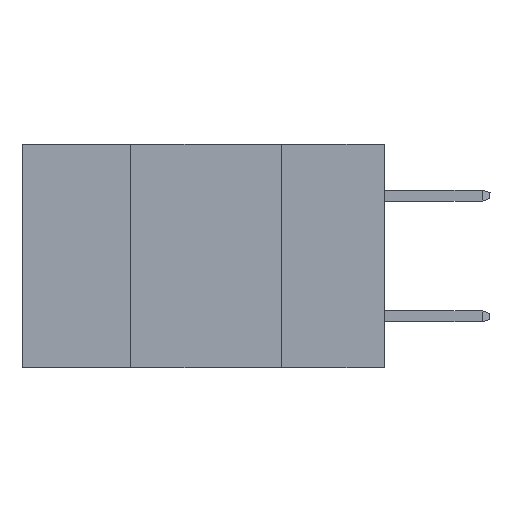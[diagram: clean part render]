
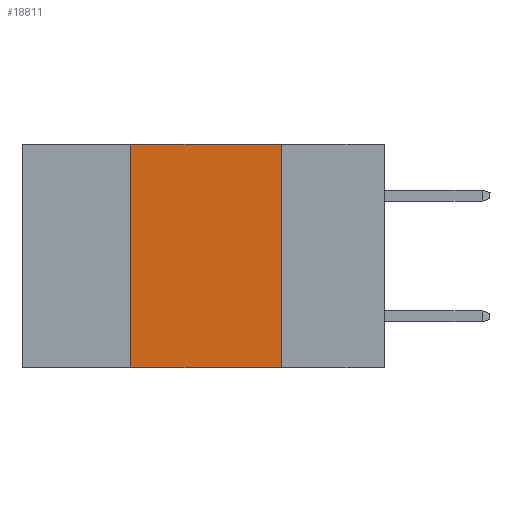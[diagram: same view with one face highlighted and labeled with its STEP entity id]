
A CAD part, left-side view. The second image highlights one B-rep face of the part: STEP entity #18811.
In plain terms, the highlighted planar face has unit normal (-1, 0, 0).
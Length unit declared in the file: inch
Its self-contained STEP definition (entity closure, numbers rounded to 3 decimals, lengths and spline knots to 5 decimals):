
#59 = ORIENTED_EDGE ( 'NONE', *, *, #3938, .T. ) ;
#1179 = CARTESIAN_POINT ( 'NONE',  ( 0., 0.42, -0.37 ) ) ;
#1969 = EDGE_CURVE ( 'NONE', #14255, #6165, #17362, .T. ) ;
#2814 = CARTESIAN_POINT ( 'NONE',  ( 0., 0.17, -0.37 ) ) ;
#3074 = EDGE_LOOP ( 'NONE', ( #12767, #3984, #19502, #59 ) ) ;
#3472 = CARTESIAN_POINT ( 'NONE',  ( 0., 0.42, 0. ) ) ;
#3938 = EDGE_CURVE ( 'NONE', #10778, #6165, #16680, .T. ) ;
#3984 = ORIENTED_EDGE ( 'NONE', *, *, #18024, .F. ) ;
#4234 = CARTESIAN_POINT ( 'NONE',  ( 0., 0.42, -0.37 ) ) ;
#4297 = LINE ( 'NONE', #8624, #9271 ) ;
#5072 = CARTESIAN_POINT ( 'NONE',  ( 0., 0.6, 0. ) ) ;
#5873 = DIRECTION ( 'NONE',  ( 0., 0., -1. ) ) ;
#6165 = VERTEX_POINT ( 'NONE', #2814 ) ;
#6980 = DIRECTION ( 'NONE',  ( 0., 0., -1. ) ) ;
#7395 = CARTESIAN_POINT ( 'NONE',  ( 0., 0.17, -0.37 ) ) ;
#7446 = VECTOR ( 'NONE', #5873, 39.37008 ) ;
#8624 = CARTESIAN_POINT ( 'NONE',  ( 0., 0.6, 0. ) ) ;
#9271 = VECTOR ( 'NONE', #23554, 39.37008 ) ;
#10482 = EDGE_CURVE ( 'NONE', #10778, #23577, #22296, .T. ) ;
#10568 = AXIS2_PLACEMENT_3D ( 'NONE', #5072, #18155, #6980 ) ;
#10778 = VERTEX_POINT ( 'NONE', #1179 ) ;
#11754 = VECTOR ( 'NONE', #21077, 39.37008 ) ;
#12767 = ORIENTED_EDGE ( 'NONE', *, *, #1969, .F. ) ;
#14255 = VERTEX_POINT ( 'NONE', #22399 ) ;
#15574 = DIRECTION ( 'NONE',  ( 0., -1., 0. ) ) ;
#15597 = CARTESIAN_POINT ( 'NONE',  ( 0., 0.6, -0.37 ) ) ;
#16680 = LINE ( 'NONE', #15597, #19879 ) ;
#17362 = LINE ( 'NONE', #7395, #7446 ) ;
#18024 = EDGE_CURVE ( 'NONE', #23577, #14255, #4297, .T. ) ;
#18155 = DIRECTION ( 'NONE',  ( 1., 0., 0. ) ) ;
#18811 = ADVANCED_FACE ( 'NONE', ( #21831 ), #21798, .F. ) ;
#19502 = ORIENTED_EDGE ( 'NONE', *, *, #10482, .F. ) ;
#19879 = VECTOR ( 'NONE', #15574, 39.37008 ) ;
#21077 = DIRECTION ( 'NONE',  ( 0., 0., 1. ) ) ;
#21798 = PLANE ( 'NONE',  #10568 ) ;
#21831 = FACE_OUTER_BOUND ( 'NONE', #3074, .T. ) ;
#22296 = LINE ( 'NONE', #4234, #11754 ) ;
#22399 = CARTESIAN_POINT ( 'NONE',  ( 0., 0.17, 0. ) ) ;
#23554 = DIRECTION ( 'NONE',  ( 0., -1., 0. ) ) ;
#23577 = VERTEX_POINT ( 'NONE', #3472 ) ;
